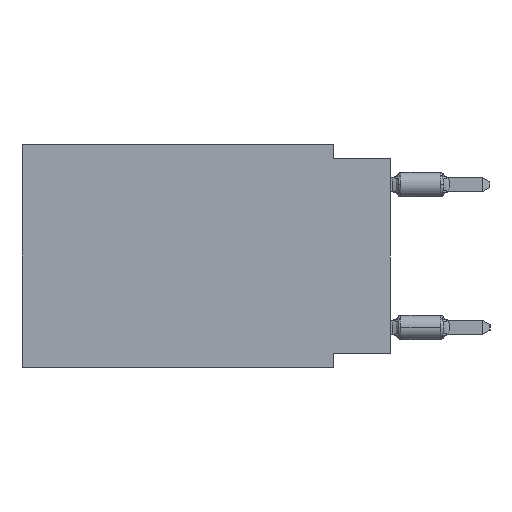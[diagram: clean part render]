
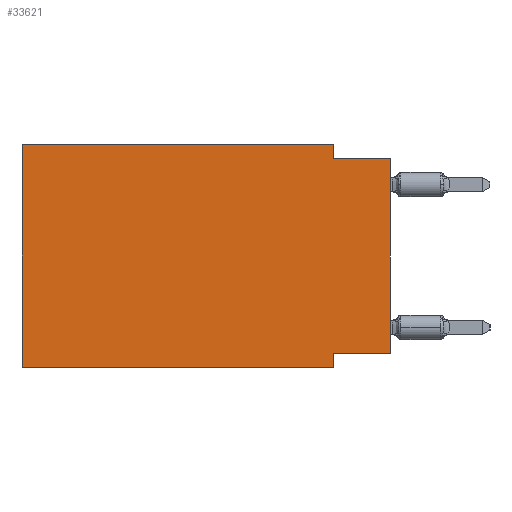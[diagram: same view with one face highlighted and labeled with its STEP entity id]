
A CAD part, left-side view. The second image highlights one B-rep face of the part: STEP entity #33621.
In plain terms, the highlighted planar face has unit normal (-1, 0, 0).
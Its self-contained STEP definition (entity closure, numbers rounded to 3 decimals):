
#164 = CARTESIAN_POINT ( 'NONE',  ( 0., 2.54, -9.906 ) ) ;
#415 = DIRECTION ( 'NONE',  ( 0., 0., 1. ) ) ;
#1053 = CARTESIAN_POINT ( 'NONE',  ( 0., 0., -0.635 ) ) ;
#1393 = EDGE_CURVE ( 'NONE', #61391, #35034, #2852, .T. ) ;
#1442 = FACE_OUTER_BOUND ( 'NONE', #36506, .T. ) ;
#2846 = AXIS2_PLACEMENT_3D ( 'NONE', #29672, #6160, #6761 ) ;
#2852 = LINE ( 'NONE', #16651, #23851 ) ;
#5767 = LINE ( 'NONE', #1053, #11367 ) ;
#6065 = CARTESIAN_POINT ( 'NONE',  ( 0., 16.383, -9.906 ) ) ;
#6160 = DIRECTION ( 'NONE',  ( 1., 0., 0. ) ) ;
#6166 = ORIENTED_EDGE ( 'NONE', *, *, #1393, .T. ) ;
#6499 = VERTEX_POINT ( 'NONE', #56071 ) ;
#6581 = VERTEX_POINT ( 'NONE', #55758 ) ;
#6761 = DIRECTION ( 'NONE',  ( 0., 0., -1. ) ) ;
#6765 = EDGE_CURVE ( 'NONE', #61391, #51895, #36040, .T. ) ;
#6869 = VERTEX_POINT ( 'NONE', #33180 ) ;
#7417 = EDGE_CURVE ( 'NONE', #51895, #16654, #51631, .T. ) ;
#8144 = VECTOR ( 'NONE', #415, 1000. ) ;
#8642 = DIRECTION ( 'NONE',  ( 0., 0., -1. ) ) ;
#11367 = VECTOR ( 'NONE', #20487, 1000. ) ;
#12234 = CARTESIAN_POINT ( 'NONE',  ( 0., 2.54, -9.271 ) ) ;
#13282 = LINE ( 'NONE', #60677, #27530 ) ;
#15134 = LINE ( 'NONE', #20158, #8144 ) ;
#16651 = CARTESIAN_POINT ( 'NONE',  ( 0., 0., 0. ) ) ;
#16654 = VERTEX_POINT ( 'NONE', #20257 ) ;
#17367 = VECTOR ( 'NONE', #8642, 1000. ) ;
#17566 = DIRECTION ( 'NONE',  ( 0., 0., 1. ) ) ;
#17800 = CARTESIAN_POINT ( 'NONE',  ( 0., 0., -9.271 ) ) ;
#17934 = ORIENTED_EDGE ( 'NONE', *, *, #6765, .F. ) ;
#18499 = ORIENTED_EDGE ( 'NONE', *, *, #19128, .F. ) ;
#19128 = EDGE_CURVE ( 'NONE', #6869, #6581, #13282, .T. ) ;
#20158 = CARTESIAN_POINT ( 'NONE',  ( 0., 16.383, 0. ) ) ;
#20257 = CARTESIAN_POINT ( 'NONE',  ( 0., 2.54, -9.906 ) ) ;
#20487 = DIRECTION ( 'NONE',  ( 0., -1., 0. ) ) ;
#21355 = CARTESIAN_POINT ( 'NONE',  ( 0., 0., -9.271 ) ) ;
#23851 = VECTOR ( 'NONE', #17566, 1000. ) ;
#26380 = EDGE_CURVE ( 'NONE', #6581, #6499, #60510, .T. ) ;
#26816 = ORIENTED_EDGE ( 'NONE', *, *, #51345, .F. ) ;
#27530 = VECTOR ( 'NONE', #61289, 1000. ) ;
#28716 = EDGE_CURVE ( 'NONE', #44461, #6869, #15134, .T. ) ;
#29672 = CARTESIAN_POINT ( 'NONE',  ( 0., 16.383, 0. ) ) ;
#32806 = CARTESIAN_POINT ( 'NONE',  ( 0., 16.383, -9.906 ) ) ;
#33008 = CARTESIAN_POINT ( 'NONE',  ( 0., 0., -0.635 ) ) ;
#33180 = CARTESIAN_POINT ( 'NONE',  ( 0., 16.383, 0. ) ) ;
#33621 = ADVANCED_FACE ( 'NONE', ( #1442 ), #45347, .F. ) ;
#35034 = VERTEX_POINT ( 'NONE', #33008 ) ;
#36040 = LINE ( 'NONE', #17800, #41188 ) ;
#36506 = EDGE_LOOP ( 'NONE', ( #6166, #26816, #42986, #18499, #49195, #37935, #41431, #17934 ) ) ;
#37529 = LINE ( 'NONE', #32806, #54753 ) ;
#37935 = ORIENTED_EDGE ( 'NONE', *, *, #45622, .T. ) ;
#41188 = VECTOR ( 'NONE', #56096, 1000. ) ;
#41431 = ORIENTED_EDGE ( 'NONE', *, *, #7417, .F. ) ;
#41683 = DIRECTION ( 'NONE',  ( 0., 0., -1. ) ) ;
#42986 = ORIENTED_EDGE ( 'NONE', *, *, #26380, .F. ) ;
#44461 = VERTEX_POINT ( 'NONE', #6065 ) ;
#45347 = PLANE ( 'NONE',  #2846 ) ;
#45622 = EDGE_CURVE ( 'NONE', #44461, #16654, #37529, .T. ) ;
#49195 = ORIENTED_EDGE ( 'NONE', *, *, #28716, .F. ) ;
#51345 = EDGE_CURVE ( 'NONE', #6499, #35034, #5767, .T. ) ;
#51404 = CARTESIAN_POINT ( 'NONE',  ( 0., 2.54, 0. ) ) ;
#51631 = LINE ( 'NONE', #164, #17367 ) ;
#51895 = VERTEX_POINT ( 'NONE', #12234 ) ;
#52123 = VECTOR ( 'NONE', #41683, 1000. ) ;
#54753 = VECTOR ( 'NONE', #56352, 1000. ) ;
#55758 = CARTESIAN_POINT ( 'NONE',  ( 0., 2.54, 0. ) ) ;
#56071 = CARTESIAN_POINT ( 'NONE',  ( 0., 2.54, -0.635 ) ) ;
#56096 = DIRECTION ( 'NONE',  ( 0., 1., 0. ) ) ;
#56352 = DIRECTION ( 'NONE',  ( 0., -1., 0. ) ) ;
#60510 = LINE ( 'NONE', #51404, #52123 ) ;
#60677 = CARTESIAN_POINT ( 'NONE',  ( 0., 16.383, 0. ) ) ;
#61289 = DIRECTION ( 'NONE',  ( 0., -1., 0. ) ) ;
#61391 = VERTEX_POINT ( 'NONE', #21355 ) ;
